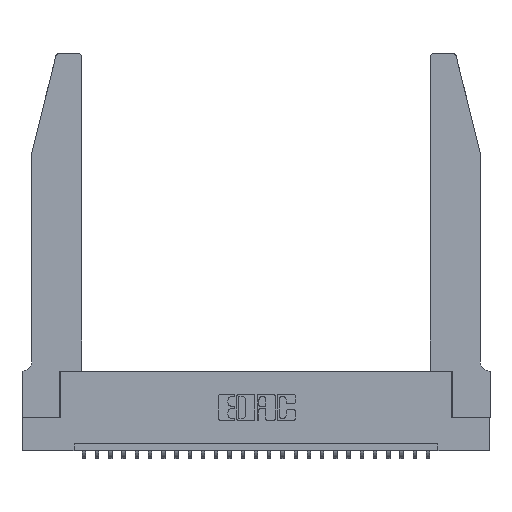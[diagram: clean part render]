
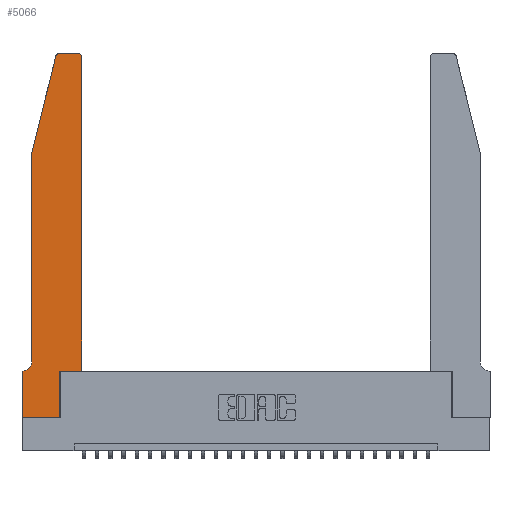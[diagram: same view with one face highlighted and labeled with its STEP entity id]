
A CAD part, top view. The second image highlights one B-rep face of the part: STEP entity #5066.
In plain terms, the highlighted planar face has unit normal (0, 0, 1).
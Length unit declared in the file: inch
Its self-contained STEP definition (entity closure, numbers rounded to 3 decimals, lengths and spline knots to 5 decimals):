
#137 = VERTEX_POINT ( 'NONE', #18081 ) ;
#737 = VERTEX_POINT ( 'NONE', #25839 ) ;
#763 = CARTESIAN_POINT ( 'NONE',  ( 0.284, 2.75, 0.37 ) ) ;
#769 = LINE ( 'NONE', #22557, #6339 ) ;
#1028 = VERTEX_POINT ( 'NONE', #13171 ) ;
#1132 = CIRCLE ( 'NONE', #21277, 0.03 ) ;
#1401 = DIRECTION ( 'NONE',  ( -1., 0., 0. ) ) ;
#1928 = LINE ( 'NONE', #12760, #17640 ) ;
#1987 = EDGE_CURVE ( 'NONE', #16681, #4560, #4021, .T. ) ;
#2381 = CARTESIAN_POINT ( 'NONE',  ( 0., 0., 0.37 ) ) ;
#3234 = CARTESIAN_POINT ( 'NONE',  ( 0., 0., 0.37 ) ) ;
#3424 = VERTEX_POINT ( 'NONE', #11893 ) ;
#4021 = CIRCLE ( 'NONE', #16815, 0.03 ) ;
#4091 = VECTOR ( 'NONE', #24186, 39.37008 ) ;
#4560 = VERTEX_POINT ( 'NONE', #8423 ) ;
#4607 = ORIENTED_EDGE ( 'NONE', *, *, #19372, .T. ) ;
#4753 = EDGE_CURVE ( 'NONE', #10083, #19607, #25480, .T. ) ;
#5066 = ADVANCED_FACE ( 'NONE', ( #9092 ), #22361, .T. ) ;
#5335 = DIRECTION ( 'NONE',  ( 0., 0., -1. ) ) ;
#5466 = DIRECTION ( 'NONE',  ( 0., -1., 0. ) ) ;
#5546 = CARTESIAN_POINT ( 'NONE',  ( 0.284, 2.72, 0.37 ) ) ;
#5706 = CARTESIAN_POINT ( 'NONE',  ( 0.2865, 0.35, 0.37 ) ) ;
#5712 = CARTESIAN_POINT ( 'NONE',  ( 0.4505, 2.72, 0.37 ) ) ;
#6271 = CARTESIAN_POINT ( 'NONE',  ( 0., 0.35, 0.37 ) ) ;
#6339 = VECTOR ( 'NONE', #1401, 39.37008 ) ;
#6355 = EDGE_CURVE ( 'NONE', #1028, #18629, #11277, .T. ) ;
#6615 = DIRECTION ( 'NONE',  ( -1., 0., 0. ) ) ;
#6898 = DIRECTION ( 'NONE',  ( 0., 1., 0. ) ) ;
#7025 = VECTOR ( 'NONE', #5466, 39.37008 ) ;
#7071 = DIRECTION ( 'NONE',  ( 0., -1., 0. ) ) ;
#7199 = CIRCLE ( 'NONE', #7254, 0.07 ) ;
#7254 = AXIS2_PLACEMENT_3D ( 'NONE', #22188, #5335, #22091 ) ;
#7281 = VECTOR ( 'NONE', #6898, 39.37008 ) ;
#7514 = VERTEX_POINT ( 'NONE', #23925 ) ;
#7515 = EDGE_CURVE ( 'NONE', #7514, #13652, #14203, .T. ) ;
#8342 = ORIENTED_EDGE ( 'NONE', *, *, #1987, .T. ) ;
#8423 = CARTESIAN_POINT ( 'NONE',  ( 0.25487, 2.72718, 0.37 ) ) ;
#9022 = ORIENTED_EDGE ( 'NONE', *, *, #26937, .T. ) ;
#9092 = FACE_OUTER_BOUND ( 'NONE', #24924, .T. ) ;
#10083 = VERTEX_POINT ( 'NONE', #6271 ) ;
#10246 = DIRECTION ( 'NONE',  ( 1., 0., 0. ) ) ;
#11277 = LINE ( 'NONE', #5706, #4091 ) ;
#11576 = LINE ( 'NONE', #26742, #18127 ) ;
#11809 = ORIENTED_EDGE ( 'NONE', *, *, #7515, .T. ) ;
#11852 = DIRECTION ( 'NONE',  ( 0., 0., 1. ) ) ;
#11893 = CARTESIAN_POINT ( 'NONE',  ( 0.0055, 0.35, 0.37 ) ) ;
#12514 = ORIENTED_EDGE ( 'NONE', *, *, #26653, .T. ) ;
#12760 = CARTESIAN_POINT ( 'NONE',  ( 0.2605, 2.75, 0.37 ) ) ;
#13081 = VERTEX_POINT ( 'NONE', #24027 ) ;
#13171 = CARTESIAN_POINT ( 'NONE',  ( 0.2865, 0., 0.37 ) ) ;
#13412 = EDGE_CURVE ( 'NONE', #18629, #7514, #11576, .T. ) ;
#13514 = VECTOR ( 'NONE', #21239, 39.37008 ) ;
#13652 = VERTEX_POINT ( 'NONE', #5712 ) ;
#14044 = LINE ( 'NONE', #16775, #15643 ) ;
#14203 = LINE ( 'NONE', #19431, #7281 ) ;
#14973 = VECTOR ( 'NONE', #7071, 39.37008 ) ;
#15643 = VECTOR ( 'NONE', #20804, 39.37008 ) ;
#15897 = CARTESIAN_POINT ( 'NONE',  ( 0.0755, 2., 0.37 ) ) ;
#16016 = ORIENTED_EDGE ( 'NONE', *, *, #26816, .T. ) ;
#16681 = VERTEX_POINT ( 'NONE', #763 ) ;
#16775 = CARTESIAN_POINT ( 'NONE',  ( 0.0755, 2., 0.37 ) ) ;
#16815 = AXIS2_PLACEMENT_3D ( 'NONE', #5546, #20182, #17885 ) ;
#16855 = LINE ( 'NONE', #15897, #7025 ) ;
#17640 = VECTOR ( 'NONE', #6615, 39.37008 ) ;
#17885 = DIRECTION ( 'NONE',  ( 1., 0., 0. ) ) ;
#18081 = CARTESIAN_POINT ( 'NONE',  ( 0.0755, 2., 0.37 ) ) ;
#18122 = CARTESIAN_POINT ( 'NONE',  ( 0., 0.35, 0.37 ) ) ;
#18127 = VECTOR ( 'NONE', #10246, 39.37008 ) ;
#18217 = DIRECTION ( 'NONE',  ( 0., 0., 1. ) ) ;
#18374 = CARTESIAN_POINT ( 'NONE',  ( 0., 0., 0.37 ) ) ;
#18629 = VERTEX_POINT ( 'NONE', #25892 ) ;
#19372 = EDGE_CURVE ( 'NONE', #13081, #3424, #7199, .T. ) ;
#19431 = CARTESIAN_POINT ( 'NONE',  ( 0.4505, 0.35, 0.37 ) ) ;
#19476 = ORIENTED_EDGE ( 'NONE', *, *, #21111, .T. ) ;
#19607 = VERTEX_POINT ( 'NONE', #18374 ) ;
#19816 = ORIENTED_EDGE ( 'NONE', *, *, #4753, .T. ) ;
#20182 = DIRECTION ( 'NONE',  ( 0., 0., 1. ) ) ;
#20737 = ORIENTED_EDGE ( 'NONE', *, *, #24113, .T. ) ;
#20804 = DIRECTION ( 'NONE',  ( -0.239, -0.971, 0. ) ) ;
#21111 = EDGE_CURVE ( 'NONE', #3424, #10083, #769, .T. ) ;
#21239 = DIRECTION ( 'NONE',  ( 1., 0., 0. ) ) ;
#21277 = AXIS2_PLACEMENT_3D ( 'NONE', #24395, #11852, #22297 ) ;
#21309 = ORIENTED_EDGE ( 'NONE', *, *, #6355, .T. ) ;
#21353 = EDGE_CURVE ( 'NONE', #19607, #1028, #24342, .T. ) ;
#22091 = DIRECTION ( 'NONE',  ( -1., 0., 0. ) ) ;
#22188 = CARTESIAN_POINT ( 'NONE',  ( 0.0055, 0.42, 0.37 ) ) ;
#22297 = DIRECTION ( 'NONE',  ( 1., 0., 0. ) ) ;
#22361 = PLANE ( 'NONE',  #24235 ) ;
#22557 = CARTESIAN_POINT ( 'NONE',  ( 0.0755, 0.35, 0.37 ) ) ;
#22628 = DIRECTION ( 'NONE',  ( 1., 0., 0. ) ) ;
#23925 = CARTESIAN_POINT ( 'NONE',  ( 0.4505, 0.35, 0.37 ) ) ;
#24027 = CARTESIAN_POINT ( 'NONE',  ( 0.0755, 0.42, 0.37 ) ) ;
#24113 = EDGE_CURVE ( 'NONE', #4560, #137, #14044, .T. ) ;
#24186 = DIRECTION ( 'NONE',  ( 0., 1., 0. ) ) ;
#24235 = AXIS2_PLACEMENT_3D ( 'NONE', #18122, #18217, #22628 ) ;
#24342 = LINE ( 'NONE', #2381, #13514 ) ;
#24395 = CARTESIAN_POINT ( 'NONE',  ( 0.4205, 2.72, 0.37 ) ) ;
#24924 = EDGE_LOOP ( 'NONE', ( #9022, #8342, #20737, #12514, #4607, #19476, #19816, #26667, #21309, #26207, #11809, #16016 ) ) ;
#25480 = LINE ( 'NONE', #3234, #14973 ) ;
#25839 = CARTESIAN_POINT ( 'NONE',  ( 0.4205, 2.75, 0.37 ) ) ;
#25892 = CARTESIAN_POINT ( 'NONE',  ( 0.2865, 0.35, 0.37 ) ) ;
#26207 = ORIENTED_EDGE ( 'NONE', *, *, #13412, .T. ) ;
#26653 = EDGE_CURVE ( 'NONE', #137, #13081, #16855, .T. ) ;
#26667 = ORIENTED_EDGE ( 'NONE', *, *, #21353, .T. ) ;
#26742 = CARTESIAN_POINT ( 'NONE',  ( 0.4505, 0.35, 0.37 ) ) ;
#26816 = EDGE_CURVE ( 'NONE', #13652, #737, #1132, .T. ) ;
#26937 = EDGE_CURVE ( 'NONE', #737, #16681, #1928, .T. ) ;
